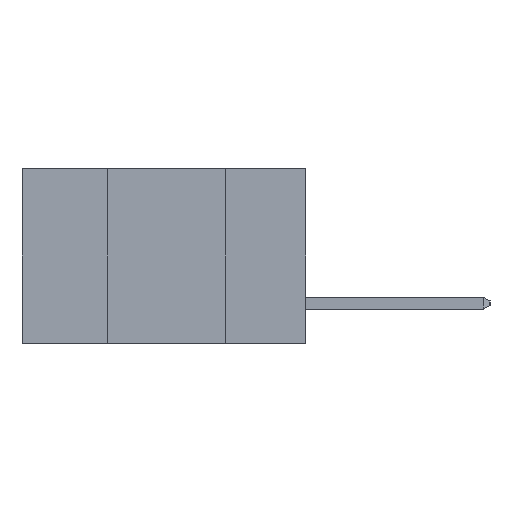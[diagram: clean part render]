
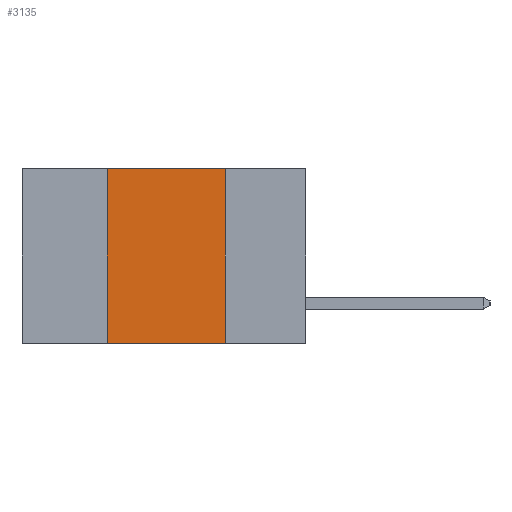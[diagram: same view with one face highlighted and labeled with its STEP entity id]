
A CAD part, left-side view. The second image highlights one B-rep face of the part: STEP entity #3135.
In plain terms, the highlighted planar face has unit normal (-1, 0, 0).
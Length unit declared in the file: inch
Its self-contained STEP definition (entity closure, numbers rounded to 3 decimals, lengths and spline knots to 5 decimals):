
#97 = EDGE_CURVE ( 'NONE', #15081, #15465, #6660, .T. ) ;
#307 = CARTESIAN_POINT ( 'NONE',  ( 0., 0.6, 0. ) ) ;
#347 = LINE ( 'NONE', #2654, #10198 ) ;
#668 = DIRECTION ( 'NONE',  ( 0., -1., 0. ) ) ;
#676 = CARTESIAN_POINT ( 'NONE',  ( 0., 0.17, -0.37 ) ) ;
#1070 = LINE ( 'NONE', #15673, #7160 ) ;
#1127 = EDGE_CURVE ( 'NONE', #12680, #2665, #347, .T. ) ;
#2565 = CARTESIAN_POINT ( 'NONE',  ( 0., 0.6, 0. ) ) ;
#2654 = CARTESIAN_POINT ( 'NONE',  ( 0., 0.6, -0.37 ) ) ;
#2665 = VERTEX_POINT ( 'NONE', #676 ) ;
#2919 = DIRECTION ( 'NONE',  ( 0., 0., -1. ) ) ;
#3135 = ADVANCED_FACE ( 'NONE', ( #7773 ), #8045, .F. ) ;
#4016 = ORIENTED_EDGE ( 'NONE', *, *, #9430, .F. ) ;
#4157 = DIRECTION ( 'NONE',  ( 0., 0., -1. ) ) ;
#5076 = ORIENTED_EDGE ( 'NONE', *, *, #14940, .F. ) ;
#5276 = CARTESIAN_POINT ( 'NONE',  ( 0., 0.42, 0. ) ) ;
#6375 = LINE ( 'NONE', #5276, #9757 ) ;
#6493 = DIRECTION ( 'NONE',  ( 0., 0., 1. ) ) ;
#6660 = LINE ( 'NONE', #2565, #16059 ) ;
#6681 = ORIENTED_EDGE ( 'NONE', *, *, #97, .F. ) ;
#7160 = VECTOR ( 'NONE', #4157, 39.37008 ) ;
#7773 = FACE_OUTER_BOUND ( 'NONE', #9259, .T. ) ;
#8045 = PLANE ( 'NONE',  #11715 ) ;
#9259 = EDGE_LOOP ( 'NONE', ( #4016, #6681, #5076, #15331 ) ) ;
#9430 = EDGE_CURVE ( 'NONE', #15465, #2665, #1070, .T. ) ;
#9757 = VECTOR ( 'NONE', #6493, 39.37008 ) ;
#10198 = VECTOR ( 'NONE', #16385, 39.37008 ) ;
#10202 = CARTESIAN_POINT ( 'NONE',  ( 0., 0.42, -0.37 ) ) ;
#10596 = DIRECTION ( 'NONE',  ( 1., 0., 0. ) ) ;
#11715 = AXIS2_PLACEMENT_3D ( 'NONE', #307, #10596, #2919 ) ;
#12680 = VERTEX_POINT ( 'NONE', #10202 ) ;
#14431 = CARTESIAN_POINT ( 'NONE',  ( 0., 0.42, 0. ) ) ;
#14940 = EDGE_CURVE ( 'NONE', #12680, #15081, #6375, .T. ) ;
#15081 = VERTEX_POINT ( 'NONE', #14431 ) ;
#15151 = CARTESIAN_POINT ( 'NONE',  ( 0., 0.17, 0. ) ) ;
#15331 = ORIENTED_EDGE ( 'NONE', *, *, #1127, .T. ) ;
#15465 = VERTEX_POINT ( 'NONE', #15151 ) ;
#15673 = CARTESIAN_POINT ( 'NONE',  ( 0., 0.17, 0. ) ) ;
#16059 = VECTOR ( 'NONE', #668, 39.37008 ) ;
#16385 = DIRECTION ( 'NONE',  ( 0., -1., 0. ) ) ;
